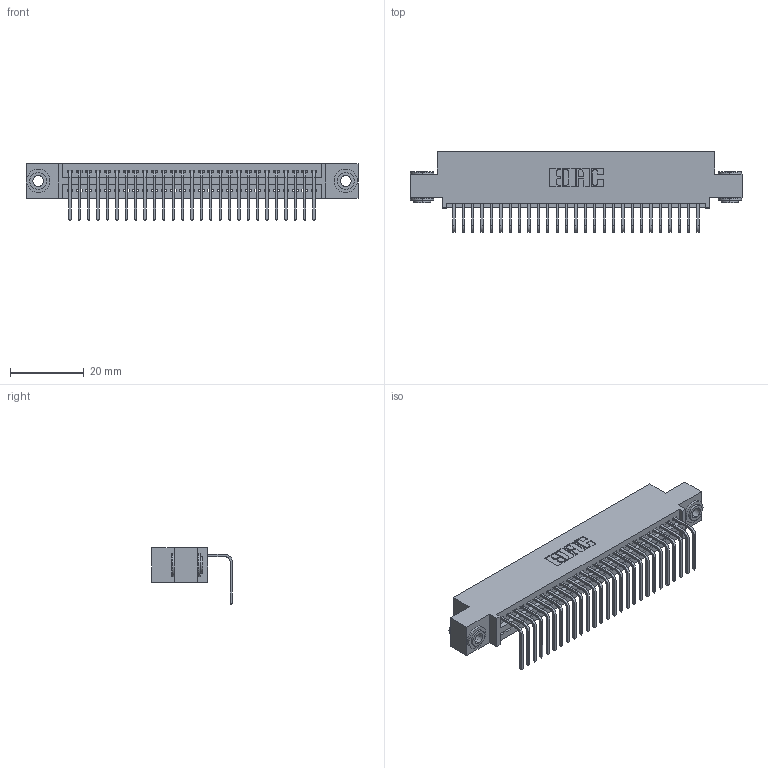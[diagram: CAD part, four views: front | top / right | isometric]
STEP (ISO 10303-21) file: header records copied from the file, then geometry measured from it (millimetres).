
FILE_DESCRIPTION (( 'STEP AP203' ), '1' );
FILE_NAME ('345-027-558-403.STEP', '2019-10-10T13:45:43', ( '' ), ( '' ), 'SwSTEP 2.0', 'SolidWorks 2016', '' );
FILE_SCHEMA (( 'CONFIG_CONTROL_DESIGN' ));
Length unit declared in the file: inch
Products named in the file (4): 345 Part_0.110 Offset - 0.156 Dia-TH; 345-292-001_558 Tail - 2; 345-250-002_345-250-002-102; 345-027-558-403
Assembly tree (30 placements, depth 2):
  345-027-558-403
    345 Part_0.110 Offset - 0.156 Dia-TH
    345-292-001_558 Tail - 2  x27
    345-250-002_345-250-002-102  x2
Bounding box: 89.79 x 21.83 x 15.37 mm (x, y, z)
Volume: 8441.4 mm3; surface area: 11838.9 mm2
Topology: 30 solids, 30 shells, 1788 faces, 5343 edges, 3522 vertices
Faces by surface type: plane 1228, cylinder 552, cone 8
Entity records: 23206 total; most frequent: CARTESIAN_POINT 4000, ORIENTED_EDGE 3954, DIRECTION 3545, EDGE_CURVE 1977, VECTOR 1713, LINE 1713, VERTEX_POINT 1314, AXIS2_PLACEMENT_3D 916
